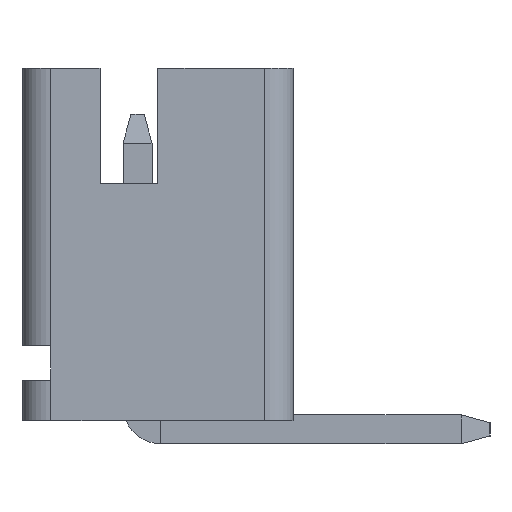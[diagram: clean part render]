
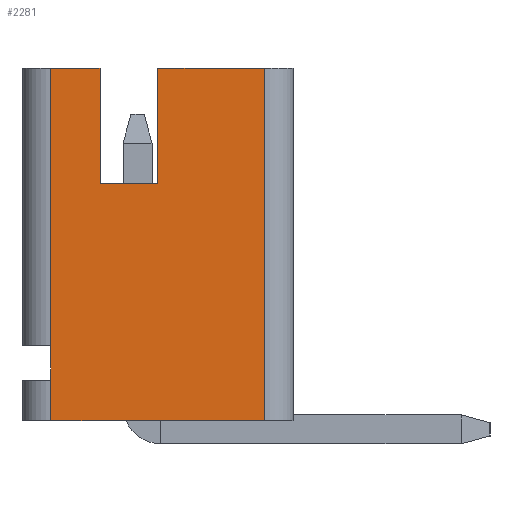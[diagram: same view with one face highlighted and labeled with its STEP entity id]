
A CAD part, left-side view. The second image highlights one B-rep face of the part: STEP entity #2281.
In plain terms, the highlighted planar face has unit normal (-1, 0, 0).
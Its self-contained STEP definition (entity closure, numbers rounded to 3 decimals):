
#38 = CARTESIAN_POINT ( 'NONE',  ( -2., -0.35, 4.1 ) ) ;
#58 = LINE ( 'NONE', #1743, #5282 ) ;
#118 = EDGE_CURVE ( 'NONE', #3417, #3711, #1042, .T. ) ;
#209 = LINE ( 'NONE', #2774, #5039 ) ;
#297 = CARTESIAN_POINT ( 'NONE',  ( -2., 2., 0. ) ) ;
#432 = CARTESIAN_POINT ( 'NONE',  ( -2., 0.65, 6.1 ) ) ;
#447 = CARTESIAN_POINT ( 'NONE',  ( -2., -2.2, 0. ) ) ;
#607 = LINE ( 'NONE', #4315, #3272 ) ;
#622 = VECTOR ( 'NONE', #3967, 1000. ) ;
#651 = DIRECTION ( 'NONE',  ( 0., 1., 0. ) ) ;
#846 = CARTESIAN_POINT ( 'NONE',  ( -2., 1.5, 6.1 ) ) ;
#895 = VERTEX_POINT ( 'NONE', #1344 ) ;
#1042 = LINE ( 'NONE', #297, #2164 ) ;
#1044 = CARTESIAN_POINT ( 'NONE',  ( -2., 1.5, 1.3 ) ) ;
#1066 = DIRECTION ( 'NONE',  ( 0., -1., 0. ) ) ;
#1146 = DIRECTION ( 'NONE',  ( 0., 0., -1. ) ) ;
#1162 = CARTESIAN_POINT ( 'NONE',  ( -2., 0., 0. ) ) ;
#1174 = ORIENTED_EDGE ( 'NONE', *, *, #2463, .T. ) ;
#1344 = CARTESIAN_POINT ( 'NONE',  ( -2., -0.35, 6.1 ) ) ;
#1387 = ORIENTED_EDGE ( 'NONE', *, *, #4384, .T. ) ;
#1420 = VECTOR ( 'NONE', #1146, 1000. ) ;
#1509 = VECTOR ( 'NONE', #4434, 1000. ) ;
#1541 = EDGE_CURVE ( 'NONE', #3256, #4731, #5336, .T. ) ;
#1567 = LINE ( 'NONE', #3246, #1420 ) ;
#1729 = CARTESIAN_POINT ( 'NONE',  ( -2., -2.2, 0. ) ) ;
#1743 = CARTESIAN_POINT ( 'NONE',  ( -2., 0.65, 6.1 ) ) ;
#1781 = CARTESIAN_POINT ( 'NONE',  ( -2., 1.5, 0. ) ) ;
#1831 = CARTESIAN_POINT ( 'NONE',  ( -2., 1.5, 1.3 ) ) ;
#1880 = EDGE_CURVE ( 'NONE', #4617, #3417, #1567, .T. ) ;
#1883 = LINE ( 'NONE', #2738, #1509 ) ;
#1931 = AXIS2_PLACEMENT_3D ( 'NONE', #1162, #2845, #2356 ) ;
#1943 = PLANE ( 'NONE',  #1931 ) ;
#1995 = FACE_OUTER_BOUND ( 'NONE', #2265, .T. ) ;
#2087 = EDGE_CURVE ( 'NONE', #895, #3256, #2856, .T. ) ;
#2096 = EDGE_CURVE ( 'NONE', #3601, #2570, #1883, .T. ) ;
#2164 = VECTOR ( 'NONE', #1066, 1000. ) ;
#2265 = EDGE_LOOP ( 'NONE', ( #5328, #3436, #2651, #5375, #2394, #1174, #4050, #3227, #1387, #3980 ) ) ;
#2281 = ADVANCED_FACE ( 'NONE', ( #1995 ), #1943, .T. ) ;
#2331 = DIRECTION ( 'NONE',  ( 0., 0., -1. ) ) ;
#2356 = DIRECTION ( 'NONE',  ( 0., -1., 0. ) ) ;
#2394 = ORIENTED_EDGE ( 'NONE', *, *, #1541, .T. ) ;
#2448 = VECTOR ( 'NONE', #4425, 1000. ) ;
#2463 = EDGE_CURVE ( 'NONE', #4731, #3288, #58, .T. ) ;
#2526 = EDGE_CURVE ( 'NONE', #2923, #895, #607, .T. ) ;
#2544 = CARTESIAN_POINT ( 'NONE',  ( -2., 1.5, 0.7 ) ) ;
#2570 = VERTEX_POINT ( 'NONE', #1044 ) ;
#2651 = ORIENTED_EDGE ( 'NONE', *, *, #2526, .T. ) ;
#2738 = CARTESIAN_POINT ( 'NONE',  ( -2., 1.5, 0. ) ) ;
#2774 = CARTESIAN_POINT ( 'NONE',  ( -2., 2., 6.1 ) ) ;
#2845 = DIRECTION ( 'NONE',  ( -1., 0., 0. ) ) ;
#2856 = LINE ( 'NONE', #4523, #622 ) ;
#2923 = VERTEX_POINT ( 'NONE', #3356 ) ;
#3065 = CARTESIAN_POINT ( 'NONE',  ( -2., 0.65, 4.1 ) ) ;
#3111 = EDGE_CURVE ( 'NONE', #3288, #3601, #209, .T. ) ;
#3227 = ORIENTED_EDGE ( 'NONE', *, *, #2096, .T. ) ;
#3246 = CARTESIAN_POINT ( 'NONE',  ( -2., 1.5, 0. ) ) ;
#3256 = VERTEX_POINT ( 'NONE', #38 ) ;
#3272 = VECTOR ( 'NONE', #3985, 1000. ) ;
#3280 = CARTESIAN_POINT ( 'NONE',  ( -2., 0.65, 4.1 ) ) ;
#3288 = VERTEX_POINT ( 'NONE', #432 ) ;
#3356 = CARTESIAN_POINT ( 'NONE',  ( -2., -2.2, 6.1 ) ) ;
#3415 = DIRECTION ( 'NONE',  ( 0., 0., 1. ) ) ;
#3417 = VERTEX_POINT ( 'NONE', #1781 ) ;
#3436 = ORIENTED_EDGE ( 'NONE', *, *, #4681, .T. ) ;
#3601 = VERTEX_POINT ( 'NONE', #846 ) ;
#3711 = VERTEX_POINT ( 'NONE', #1729 ) ;
#3796 = LINE ( 'NONE', #447, #4350 ) ;
#3829 = VECTOR ( 'NONE', #2331, 1000. ) ;
#3967 = DIRECTION ( 'NONE',  ( 0., 0., -1. ) ) ;
#3980 = ORIENTED_EDGE ( 'NONE', *, *, #1880, .T. ) ;
#3985 = DIRECTION ( 'NONE',  ( 0., 1., 0. ) ) ;
#4050 = ORIENTED_EDGE ( 'NONE', *, *, #3111, .T. ) ;
#4315 = CARTESIAN_POINT ( 'NONE',  ( -2., -0.35, 6.1 ) ) ;
#4350 = VECTOR ( 'NONE', #4675, 1000. ) ;
#4384 = EDGE_CURVE ( 'NONE', #2570, #4617, #5231, .T. ) ;
#4425 = DIRECTION ( 'NONE',  ( 0., 1., 0. ) ) ;
#4434 = DIRECTION ( 'NONE',  ( 0., 0., -1. ) ) ;
#4523 = CARTESIAN_POINT ( 'NONE',  ( -2., -0.35, 6.1 ) ) ;
#4617 = VERTEX_POINT ( 'NONE', #2544 ) ;
#4675 = DIRECTION ( 'NONE',  ( 0., 0., 1. ) ) ;
#4681 = EDGE_CURVE ( 'NONE', #3711, #2923, #3796, .T. ) ;
#4731 = VERTEX_POINT ( 'NONE', #3065 ) ;
#5039 = VECTOR ( 'NONE', #651, 1000. ) ;
#5231 = LINE ( 'NONE', #1831, #3829 ) ;
#5282 = VECTOR ( 'NONE', #3415, 1000. ) ;
#5328 = ORIENTED_EDGE ( 'NONE', *, *, #118, .T. ) ;
#5336 = LINE ( 'NONE', #3280, #2448 ) ;
#5375 = ORIENTED_EDGE ( 'NONE', *, *, #2087, .T. ) ;
